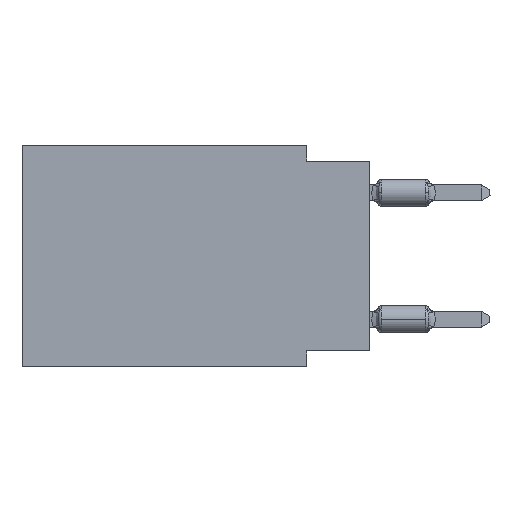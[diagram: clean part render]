
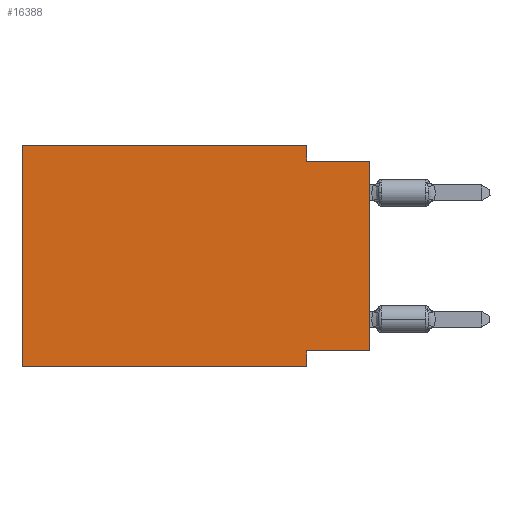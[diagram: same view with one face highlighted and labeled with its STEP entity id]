
A CAD part, left-side view. The second image highlights one B-rep face of the part: STEP entity #16388.
In plain terms, the highlighted planar face has unit normal (-1, 0, 0).
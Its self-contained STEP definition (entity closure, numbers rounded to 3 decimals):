
#494 = ORIENTED_EDGE ( 'NONE', *, *, #21888, .F. ) ;
#1279 = EDGE_CURVE ( 'NONE', #18149, #24553, #28017, .T. ) ;
#1474 = CARTESIAN_POINT ( 'NONE',  ( 0., 2.54, 0. ) ) ;
#1709 = ORIENTED_EDGE ( 'NONE', *, *, #41285, .T. ) ;
#2412 = CARTESIAN_POINT ( 'NONE',  ( 0., 2.54, -8.89 ) ) ;
#2796 = VECTOR ( 'NONE', #39703, 1000. ) ;
#3160 = VERTEX_POINT ( 'NONE', #2412 ) ;
#3234 = VERTEX_POINT ( 'NONE', #15175 ) ;
#4388 = FACE_OUTER_BOUND ( 'NONE', #9533, .T. ) ;
#4824 = LINE ( 'NONE', #1474, #2796 ) ;
#5506 = VERTEX_POINT ( 'NONE', #19450 ) ;
#5926 = EDGE_CURVE ( 'NONE', #23220, #24553, #30043, .T. ) ;
#6957 = EDGE_CURVE ( 'NONE', #32037, #19465, #21829, .T. ) ;
#8422 = EDGE_CURVE ( 'NONE', #19465, #3234, #39128, .T. ) ;
#8590 = CARTESIAN_POINT ( 'NONE',  ( 0., 13.97, 0. ) ) ;
#9533 = EDGE_LOOP ( 'NONE', ( #20629, #17234, #33370, #35352, #25055, #1709, #494, #19161 ) ) ;
#9792 = EDGE_CURVE ( 'NONE', #23220, #5506, #18287, .T. ) ;
#10367 = VECTOR ( 'NONE', #13655, 1000. ) ;
#10392 = CARTESIAN_POINT ( 'NONE',  ( 0., 13.97, -8.89 ) ) ;
#10478 = DIRECTION ( 'NONE',  ( 1., 0., 0. ) ) ;
#11399 = LINE ( 'NONE', #17649, #36956 ) ;
#12348 = CARTESIAN_POINT ( 'NONE',  ( 0., 0., -0.635 ) ) ;
#12444 = CARTESIAN_POINT ( 'NONE',  ( 0., 0., -8.255 ) ) ;
#12548 = DIRECTION ( 'NONE',  ( 0., -1., 0. ) ) ;
#12988 = DIRECTION ( 'NONE',  ( 0., 0., -1. ) ) ;
#13655 = DIRECTION ( 'NONE',  ( 0., -1., 0. ) ) ;
#13957 = AXIS2_PLACEMENT_3D ( 'NONE', #29897, #10478, #12988 ) ;
#14702 = CARTESIAN_POINT ( 'NONE',  ( 0., 0., -8.255 ) ) ;
#15175 = CARTESIAN_POINT ( 'NONE',  ( 0., 2.54, 0. ) ) ;
#15939 = VECTOR ( 'NONE', #12548, 1000. ) ;
#16182 = VECTOR ( 'NONE', #30027, 1000. ) ;
#16388 = ADVANCED_FACE ( 'NONE', ( #4388 ), #26144, .F. ) ;
#16841 = LINE ( 'NONE', #10392, #16182 ) ;
#17234 = ORIENTED_EDGE ( 'NONE', *, *, #1279, .F. ) ;
#17649 = CARTESIAN_POINT ( 'NONE',  ( 0., 2.54, -8.89 ) ) ;
#18149 = VERTEX_POINT ( 'NONE', #30059 ) ;
#18287 = LINE ( 'NONE', #12444, #18447 ) ;
#18447 = VECTOR ( 'NONE', #37696, 1000. ) ;
#19161 = ORIENTED_EDGE ( 'NONE', *, *, #9792, .F. ) ;
#19273 = EDGE_CURVE ( 'NONE', #3234, #18149, #4824, .T. ) ;
#19450 = CARTESIAN_POINT ( 'NONE',  ( 0., 2.54, -8.255 ) ) ;
#19465 = VERTEX_POINT ( 'NONE', #8590 ) ;
#20629 = ORIENTED_EDGE ( 'NONE', *, *, #5926, .T. ) ;
#21829 = LINE ( 'NONE', #22232, #22949 ) ;
#21888 = EDGE_CURVE ( 'NONE', #5506, #3160, #11399, .T. ) ;
#22052 = CARTESIAN_POINT ( 'NONE',  ( 0., 13.97, -8.89 ) ) ;
#22232 = CARTESIAN_POINT ( 'NONE',  ( 0., 13.97, 0. ) ) ;
#22448 = DIRECTION ( 'NONE',  ( 0., 0., 1. ) ) ;
#22949 = VECTOR ( 'NONE', #22448, 1000. ) ;
#23220 = VERTEX_POINT ( 'NONE', #14702 ) ;
#23482 = CARTESIAN_POINT ( 'NONE',  ( 0., 13.97, 0. ) ) ;
#24210 = VECTOR ( 'NONE', #27539, 1000. ) ;
#24339 = DIRECTION ( 'NONE',  ( 0., 0., -1. ) ) ;
#24553 = VERTEX_POINT ( 'NONE', #35146 ) ;
#25055 = ORIENTED_EDGE ( 'NONE', *, *, #6957, .F. ) ;
#26144 = PLANE ( 'NONE',  #13957 ) ;
#27539 = DIRECTION ( 'NONE',  ( 0., 0., 1. ) ) ;
#28017 = LINE ( 'NONE', #12348, #15939 ) ;
#29897 = CARTESIAN_POINT ( 'NONE',  ( 0., 13.97, 0. ) ) ;
#30027 = DIRECTION ( 'NONE',  ( 0., -1., 0. ) ) ;
#30043 = LINE ( 'NONE', #33773, #24210 ) ;
#30059 = CARTESIAN_POINT ( 'NONE',  ( 0., 2.54, -0.635 ) ) ;
#32037 = VERTEX_POINT ( 'NONE', #22052 ) ;
#33370 = ORIENTED_EDGE ( 'NONE', *, *, #19273, .F. ) ;
#33773 = CARTESIAN_POINT ( 'NONE',  ( 0., 0., 0. ) ) ;
#35146 = CARTESIAN_POINT ( 'NONE',  ( 0., 0., -0.635 ) ) ;
#35352 = ORIENTED_EDGE ( 'NONE', *, *, #8422, .F. ) ;
#36956 = VECTOR ( 'NONE', #24339, 1000. ) ;
#37696 = DIRECTION ( 'NONE',  ( 0., 1., 0. ) ) ;
#39128 = LINE ( 'NONE', #23482, #10367 ) ;
#39703 = DIRECTION ( 'NONE',  ( 0., 0., -1. ) ) ;
#41285 = EDGE_CURVE ( 'NONE', #32037, #3160, #16841, .T. ) ;
